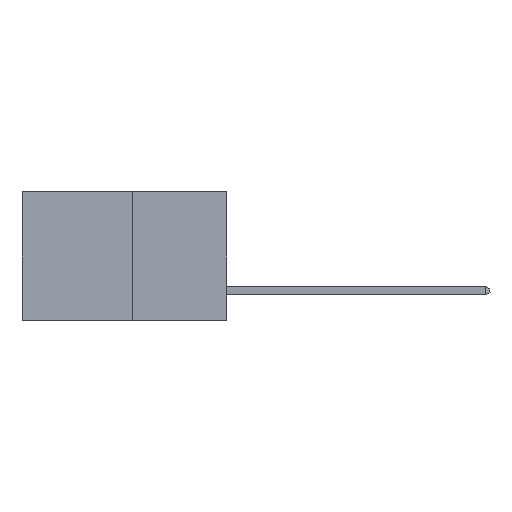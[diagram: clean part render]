
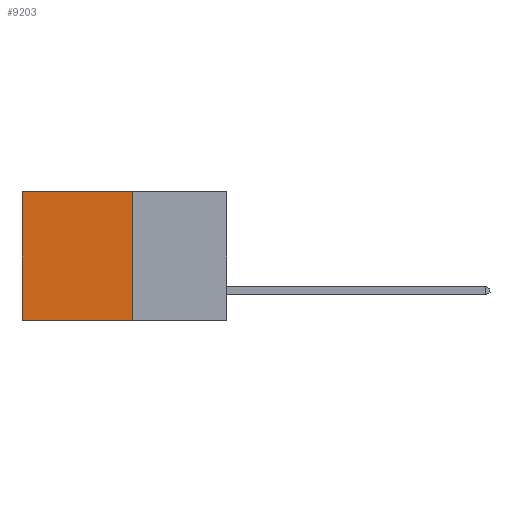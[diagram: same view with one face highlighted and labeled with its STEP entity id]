
A CAD part, left-side view. The second image highlights one B-rep face of the part: STEP entity #9203.
In plain terms, the highlighted planar face has unit normal (-1, 0, 0).
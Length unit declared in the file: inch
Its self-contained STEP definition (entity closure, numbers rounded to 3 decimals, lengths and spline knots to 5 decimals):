
#10 = CARTESIAN_POINT ( 'NONE',  ( 0.277, 0.27, 0. ) ) ;
#17 = AXIS2_PLACEMENT_3D ( 'NONE', #5492, #6217, #1750 ) ;
#159 = PLANE ( 'NONE',  #17 ) ;
#278 = VERTEX_POINT ( 'NONE', #1884 ) ;
#426 = VERTEX_POINT ( 'NONE', #2608 ) ;
#1352 = ORIENTED_EDGE ( 'NONE', *, *, #5839, .F. ) ;
#1750 = DIRECTION ( 'NONE',  ( 0., 0., -1. ) ) ;
#1884 = CARTESIAN_POINT ( 'NONE',  ( 0.277, 0.27, -0.37 ) ) ;
#2089 = ORIENTED_EDGE ( 'NONE', *, *, #5106, .T. ) ;
#2493 = EDGE_CURVE ( 'NONE', #2759, #278, #6491, .T. ) ;
#2608 = CARTESIAN_POINT ( 'NONE',  ( 0.277, 0.59, 0. ) ) ;
#2759 = VERTEX_POINT ( 'NONE', #9256 ) ;
#2924 = ORIENTED_EDGE ( 'NONE', *, *, #5882, .T. ) ;
#3747 = FACE_OUTER_BOUND ( 'NONE', #6584, .T. ) ;
#4014 = CARTESIAN_POINT ( 'NONE',  ( 0.277, 0.27, -0.37 ) ) ;
#4234 = DIRECTION ( 'NONE',  ( 0., 0., -1. ) ) ;
#4597 = CARTESIAN_POINT ( 'NONE',  ( 0.277, 0.59, -0.37 ) ) ;
#4628 = DIRECTION ( 'NONE',  ( 0., 0., -1. ) ) ;
#4953 = DIRECTION ( 'NONE',  ( 0., 1., 0. ) ) ;
#4964 = CARTESIAN_POINT ( 'NONE',  ( 0.277, 0.27, -0.37 ) ) ;
#5027 = VECTOR ( 'NONE', #9594, 39.37008 ) ;
#5106 = EDGE_CURVE ( 'NONE', #2759, #426, #8842, .T. ) ;
#5213 = VERTEX_POINT ( 'NONE', #8944 ) ;
#5492 = CARTESIAN_POINT ( 'NONE',  ( 0.277, 0.27, -0.37 ) ) ;
#5839 = EDGE_CURVE ( 'NONE', #278, #5213, #9245, .T. ) ;
#5882 = EDGE_CURVE ( 'NONE', #426, #5213, #9038, .T. ) ;
#6217 = DIRECTION ( 'NONE',  ( 1., 0., 0. ) ) ;
#6261 = VECTOR ( 'NONE', #4234, 39.37008 ) ;
#6491 = LINE ( 'NONE', #4014, #6261 ) ;
#6584 = EDGE_LOOP ( 'NONE', ( #2924, #1352, #7752, #2089 ) ) ;
#7148 = VECTOR ( 'NONE', #4628, 39.37008 ) ;
#7752 = ORIENTED_EDGE ( 'NONE', *, *, #2493, .F. ) ;
#8842 = LINE ( 'NONE', #10, #5027 ) ;
#8944 = CARTESIAN_POINT ( 'NONE',  ( 0.277, 0.59, -0.37 ) ) ;
#9038 = LINE ( 'NONE', #4597, #7148 ) ;
#9203 = ADVANCED_FACE ( 'NONE', ( #3747 ), #159, .F. ) ;
#9245 = LINE ( 'NONE', #4964, #9482 ) ;
#9256 = CARTESIAN_POINT ( 'NONE',  ( 0.277, 0.27, 0. ) ) ;
#9482 = VECTOR ( 'NONE', #4953, 39.37008 ) ;
#9594 = DIRECTION ( 'NONE',  ( 0., 1., 0. ) ) ;
